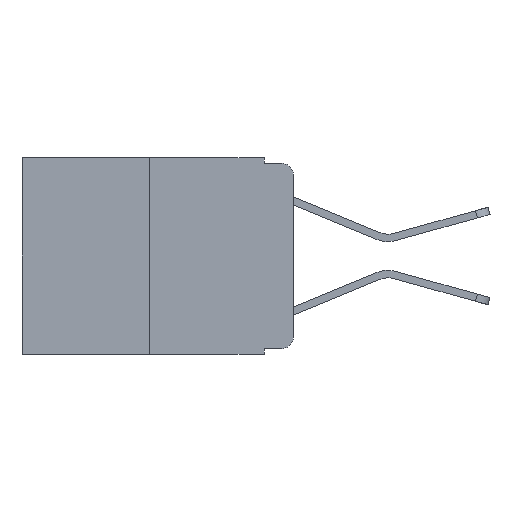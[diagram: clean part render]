
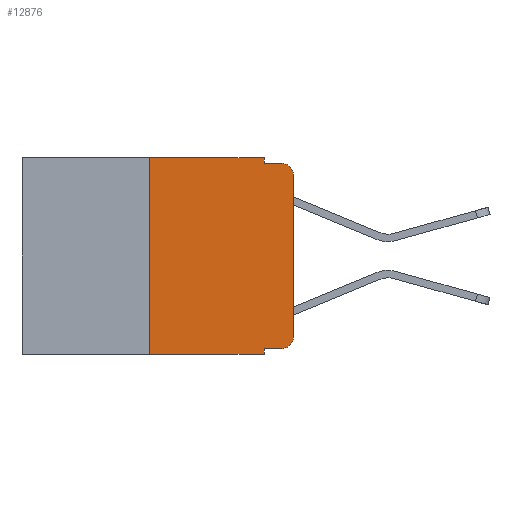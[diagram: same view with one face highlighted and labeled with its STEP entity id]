
A CAD part, left-side view. The second image highlights one B-rep face of the part: STEP entity #12876.
In plain terms, the highlighted planar face has unit normal (-1, 0, 0).
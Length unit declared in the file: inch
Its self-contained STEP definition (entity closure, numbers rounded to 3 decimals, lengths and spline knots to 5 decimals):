
#204 = VERTEX_POINT ( 'NONE', #3850 ) ;
#219 = LINE ( 'NONE', #24453, #21652 ) ;
#731 = VERTEX_POINT ( 'NONE', #13212 ) ;
#740 = VERTEX_POINT ( 'NONE', #15740 ) ;
#1146 = VERTEX_POINT ( 'NONE', #24383 ) ;
#1225 = CARTESIAN_POINT ( 'NONE',  ( 0., 0.051, -0.333 ) ) ;
#1489 = VECTOR ( 'NONE', #8392, 39.37008 ) ;
#1835 = VERTEX_POINT ( 'NONE', #2639 ) ;
#1969 = EDGE_CURVE ( 'NONE', #740, #204, #21536, .T. ) ;
#2020 = VERTEX_POINT ( 'NONE', #3672 ) ;
#2399 = CARTESIAN_POINT ( 'NONE',  ( 0., 0.02, -0.333 ) ) ;
#2639 = CARTESIAN_POINT ( 'NONE',  ( 0., 0., -0.03 ) ) ;
#2985 = VERTEX_POINT ( 'NONE', #8868 ) ;
#3417 = EDGE_CURVE ( 'NONE', #2020, #1146, #7167, .T. ) ;
#3672 = CARTESIAN_POINT ( 'NONE',  ( 0., 0.25, -0.343 ) ) ;
#3850 = CARTESIAN_POINT ( 'NONE',  ( 0., 0.051, -0.343 ) ) ;
#4107 = DIRECTION ( 'NONE',  ( 1., 0., 0. ) ) ;
#4205 = VECTOR ( 'NONE', #13789, 39.37008 ) ;
#4753 = DIRECTION ( 'NONE',  ( 0., 0., 1. ) ) ;
#4878 = EDGE_CURVE ( 'NONE', #2985, #7123, #12279, .T. ) ;
#5873 = DIRECTION ( 'NONE',  ( 0., 0., -1. ) ) ;
#6315 = EDGE_CURVE ( 'NONE', #7123, #731, #12199, .T. ) ;
#7123 = VERTEX_POINT ( 'NONE', #19462 ) ;
#7167 = LINE ( 'NONE', #25048, #22101 ) ;
#7258 = DIRECTION ( 'NONE',  ( 0., -1., 0. ) ) ;
#7826 = EDGE_LOOP ( 'NONE', ( #19608, #25180, #24622, #26233, #17237, #24571, #17769, #12616, #8467, #22102 ) ) ;
#7908 = EDGE_CURVE ( 'NONE', #1146, #2985, #219, .T. ) ;
#8046 = AXIS2_PLACEMENT_3D ( 'NONE', #16459, #4107, #18504 ) ;
#8198 = CARTESIAN_POINT ( 'NONE',  ( 0., 0.02, -0.03 ) ) ;
#8282 = PLANE ( 'NONE',  #8046 ) ;
#8392 = DIRECTION ( 'NONE',  ( 0., 0., 1. ) ) ;
#8467 = ORIENTED_EDGE ( 'NONE', *, *, #25870, .T. ) ;
#8582 = CIRCLE ( 'NONE', #21056, 0.02 ) ;
#8739 = DIRECTION ( 'NONE',  ( -1., 0., 0. ) ) ;
#8868 = CARTESIAN_POINT ( 'NONE',  ( 0., 0.051, 0. ) ) ;
#9107 = EDGE_CURVE ( 'NONE', #1835, #731, #8582, .T. ) ;
#9468 = EDGE_CURVE ( 'NONE', #2020, #204, #11774, .T. ) ;
#10245 = DIRECTION ( 'NONE',  ( 0., 0., -1. ) ) ;
#10340 = DIRECTION ( 'NONE',  ( 0., -1., 0. ) ) ;
#10460 = EDGE_CURVE ( 'NONE', #11606, #1835, #23394, .T. ) ;
#10784 = VECTOR ( 'NONE', #5873, 39.37008 ) ;
#11606 = VERTEX_POINT ( 'NONE', #12633 ) ;
#11774 = LINE ( 'NONE', #15371, #26587 ) ;
#12199 = LINE ( 'NONE', #22670, #22310 ) ;
#12279 = LINE ( 'NONE', #25705, #22382 ) ;
#12616 = ORIENTED_EDGE ( 'NONE', *, *, #1969, .F. ) ;
#12633 = CARTESIAN_POINT ( 'NONE',  ( 0., 0., -0.313 ) ) ;
#12876 = ADVANCED_FACE ( 'NONE', ( #19429 ), #8282, .F. ) ;
#13212 = CARTESIAN_POINT ( 'NONE',  ( 0., 0.02, -0.01 ) ) ;
#13314 = LINE ( 'NONE', #1225, #4205 ) ;
#13789 = DIRECTION ( 'NONE',  ( 0., -1., 0. ) ) ;
#14433 = CARTESIAN_POINT ( 'NONE',  ( 0., 0., 0. ) ) ;
#15371 = CARTESIAN_POINT ( 'NONE',  ( 0., 0.473, -0.343 ) ) ;
#15740 = CARTESIAN_POINT ( 'NONE',  ( 0., 0.051, -0.333 ) ) ;
#16459 = CARTESIAN_POINT ( 'NONE',  ( 0., 0.473, 0. ) ) ;
#16716 = AXIS2_PLACEMENT_3D ( 'NONE', #20883, #8739, #22906 ) ;
#16791 = CIRCLE ( 'NONE', #16716, 0.02 ) ;
#17237 = ORIENTED_EDGE ( 'NONE', *, *, #7908, .F. ) ;
#17650 = CARTESIAN_POINT ( 'NONE',  ( 0., 0.051, 0. ) ) ;
#17723 = DIRECTION ( 'NONE',  ( 0., 0., -1. ) ) ;
#17769 = ORIENTED_EDGE ( 'NONE', *, *, #9468, .T. ) ;
#18504 = DIRECTION ( 'NONE',  ( 0., 0., -1. ) ) ;
#19429 = FACE_OUTER_BOUND ( 'NONE', #7826, .T. ) ;
#19462 = CARTESIAN_POINT ( 'NONE',  ( 0., 0.051, -0.01 ) ) ;
#19608 = ORIENTED_EDGE ( 'NONE', *, *, #10460, .T. ) ;
#20883 = CARTESIAN_POINT ( 'NONE',  ( 0., 0.02, -0.313 ) ) ;
#21056 = AXIS2_PLACEMENT_3D ( 'NONE', #8198, #22364, #10245 ) ;
#21536 = LINE ( 'NONE', #17650, #10784 ) ;
#21652 = VECTOR ( 'NONE', #10340, 39.37008 ) ;
#22101 = VECTOR ( 'NONE', #4753, 39.37008 ) ;
#22102 = ORIENTED_EDGE ( 'NONE', *, *, #23170, .T. ) ;
#22310 = VECTOR ( 'NONE', #24660, 39.37008 ) ;
#22364 = DIRECTION ( 'NONE',  ( -1., 0., 0. ) ) ;
#22382 = VECTOR ( 'NONE', #17723, 39.37008 ) ;
#22670 = CARTESIAN_POINT ( 'NONE',  ( 0., 0.051, -0.01 ) ) ;
#22906 = DIRECTION ( 'NONE',  ( 0., 0., -1. ) ) ;
#23170 = EDGE_CURVE ( 'NONE', #23224, #11606, #16791, .T. ) ;
#23224 = VERTEX_POINT ( 'NONE', #2399 ) ;
#23394 = LINE ( 'NONE', #14433, #1489 ) ;
#24383 = CARTESIAN_POINT ( 'NONE',  ( 0., 0.25, 0. ) ) ;
#24453 = CARTESIAN_POINT ( 'NONE',  ( 0., 0.473, 0. ) ) ;
#24571 = ORIENTED_EDGE ( 'NONE', *, *, #3417, .F. ) ;
#24622 = ORIENTED_EDGE ( 'NONE', *, *, #6315, .F. ) ;
#24660 = DIRECTION ( 'NONE',  ( 0., -1., 0. ) ) ;
#25048 = CARTESIAN_POINT ( 'NONE',  ( 0., 0.25, 0. ) ) ;
#25180 = ORIENTED_EDGE ( 'NONE', *, *, #9107, .T. ) ;
#25705 = CARTESIAN_POINT ( 'NONE',  ( 0., 0.051, 0. ) ) ;
#25870 = EDGE_CURVE ( 'NONE', #740, #23224, #13314, .T. ) ;
#26233 = ORIENTED_EDGE ( 'NONE', *, *, #4878, .F. ) ;
#26587 = VECTOR ( 'NONE', #7258, 39.37008 ) ;
